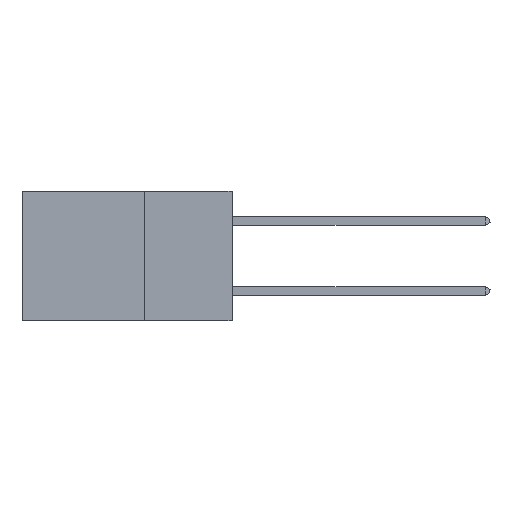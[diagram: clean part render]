
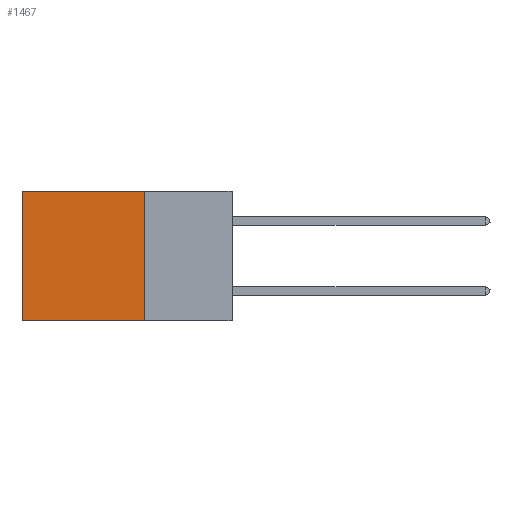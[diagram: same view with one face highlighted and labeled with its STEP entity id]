
A CAD part, left-side view. The second image highlights one B-rep face of the part: STEP entity #1467.
In plain terms, the highlighted planar face has unit normal (-1, 0, 0).
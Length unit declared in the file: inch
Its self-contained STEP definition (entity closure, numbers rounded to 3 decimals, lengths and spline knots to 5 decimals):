
#266 = DIRECTION ( 'NONE',  ( 0., 1., 0. ) ) ;
#1368 = CARTESIAN_POINT ( 'NONE',  ( 0.2875, 0.25, 0. ) ) ;
#1467 = ADVANCED_FACE ( 'NONE', ( #30150 ), #7755, .F. ) ;
#2389 = VERTEX_POINT ( 'NONE', #13491 ) ;
#2677 = CARTESIAN_POINT ( 'NONE',  ( 0.2875, 0.6, 0. ) ) ;
#5707 = VERTEX_POINT ( 'NONE', #17253 ) ;
#6812 = VECTOR ( 'NONE', #266, 39.37008 ) ;
#7246 = LINE ( 'NONE', #8618, #6812 ) ;
#7755 = PLANE ( 'NONE',  #23683 ) ;
#8618 = CARTESIAN_POINT ( 'NONE',  ( 0.2875, 0.25, 0. ) ) ;
#10323 = CARTESIAN_POINT ( 'NONE',  ( 0.2875, 0.25, -0.37 ) ) ;
#11052 = DIRECTION ( 'NONE',  ( 0., 1., 0. ) ) ;
#13491 = CARTESIAN_POINT ( 'NONE',  ( 0.2875, 0.6, -0.37 ) ) ;
#14371 = LINE ( 'NONE', #28802, #25193 ) ;
#15396 = CARTESIAN_POINT ( 'NONE',  ( 0.2875, 0.25, -0.37 ) ) ;
#16602 = EDGE_LOOP ( 'NONE', ( #23124, #32695, #21051, #21993 ) ) ;
#17253 = CARTESIAN_POINT ( 'NONE',  ( 0.2875, 0.25, 0. ) ) ;
#17693 = DIRECTION ( 'NONE',  ( 0., 0., -1. ) ) ;
#17769 = VECTOR ( 'NONE', #11052, 39.37008 ) ;
#17807 = LINE ( 'NONE', #2677, #22013 ) ;
#19325 = VERTEX_POINT ( 'NONE', #23018 ) ;
#21051 = ORIENTED_EDGE ( 'NONE', *, *, #23539, .F. ) ;
#21993 = ORIENTED_EDGE ( 'NONE', *, *, #31965, .T. ) ;
#22013 = VECTOR ( 'NONE', #17693, 39.37008 ) ;
#22280 = DIRECTION ( 'NONE',  ( 1., 0., 0. ) ) ;
#23018 = CARTESIAN_POINT ( 'NONE',  ( 0.2875, 0.6, 0. ) ) ;
#23124 = ORIENTED_EDGE ( 'NONE', *, *, #26362, .T. ) ;
#23539 = EDGE_CURVE ( 'NONE', #5707, #24054, #14371, .T. ) ;
#23683 = AXIS2_PLACEMENT_3D ( 'NONE', #1368, #22280, #31253 ) ;
#24054 = VERTEX_POINT ( 'NONE', #15396 ) ;
#25193 = VECTOR ( 'NONE', #34629, 39.37008 ) ;
#25742 = LINE ( 'NONE', #10323, #17769 ) ;
#26362 = EDGE_CURVE ( 'NONE', #19325, #2389, #17807, .T. ) ;
#26859 = EDGE_CURVE ( 'NONE', #24054, #2389, #25742, .T. ) ;
#28802 = CARTESIAN_POINT ( 'NONE',  ( 0.2875, 0.25, 0. ) ) ;
#30150 = FACE_OUTER_BOUND ( 'NONE', #16602, .T. ) ;
#31253 = DIRECTION ( 'NONE',  ( 0., 0., -1. ) ) ;
#31965 = EDGE_CURVE ( 'NONE', #5707, #19325, #7246, .T. ) ;
#32695 = ORIENTED_EDGE ( 'NONE', *, *, #26859, .F. ) ;
#34629 = DIRECTION ( 'NONE',  ( 0., 0., -1. ) ) ;
